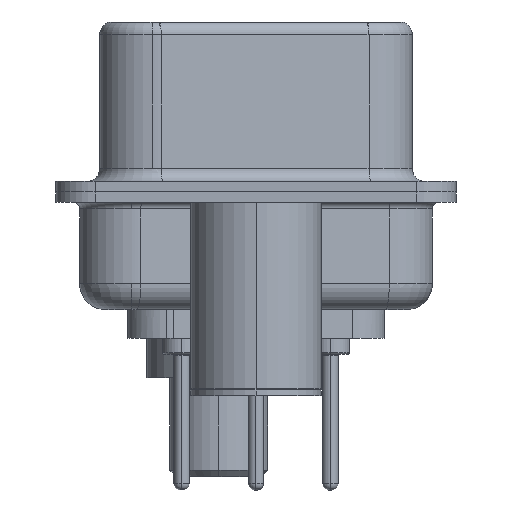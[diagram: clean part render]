
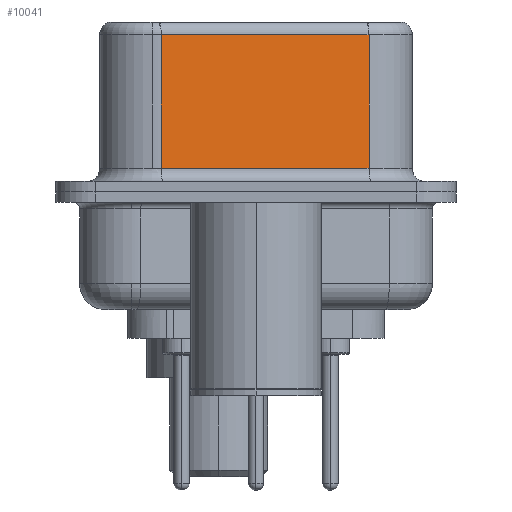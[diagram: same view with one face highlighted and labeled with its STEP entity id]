
A CAD part, left-side view. The second image highlights one B-rep face of the part: STEP entity #10041.
In plain terms, the highlighted planar face has unit normal (-0.985, -0.174, 0).
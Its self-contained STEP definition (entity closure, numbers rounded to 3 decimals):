
#919 = DIRECTION ( 'NONE',  ( 0.174, -0.985, 0. ) ) ;
#1303 = EDGE_CURVE ( 'NONE', #25222, #3450, #24702, .T. ) ;
#1446 = VERTEX_POINT ( 'NONE', #8338 ) ;
#1495 = AXIS2_PLACEMENT_3D ( 'NONE', #18260, #17339, #17264 ) ;
#2440 = VERTEX_POINT ( 'NONE', #22309 ) ;
#3299 = CARTESIAN_POINT ( 'NONE',  ( 5.132, -4.322, 0.9 ) ) ;
#3450 = VERTEX_POINT ( 'NONE', #3555 ) ;
#3555 = CARTESIAN_POINT ( 'NONE',  ( 3.73, 3.628, 0.9 ) ) ;
#4103 = LINE ( 'NONE', #16058, #23672 ) ;
#4176 = EDGE_CURVE ( 'NONE', #2440, #25222, #8430, .T. ) ;
#7643 = EDGE_CURVE ( 'NONE', #2440, #1446, #4103, .T. ) ;
#8153 = ORIENTED_EDGE ( 'NONE', *, *, #7643, .F. ) ;
#8338 = CARTESIAN_POINT ( 'NONE',  ( 5.132, -4.322, 0.9 ) ) ;
#8430 = LINE ( 'NONE', #15592, #13635 ) ;
#9150 = VECTOR ( 'NONE', #919, 1000. ) ;
#10041 = ADVANCED_FACE ( 'NONE', ( #12715 ), #17367, .F. ) ;
#10180 = DIRECTION ( 'NONE',  ( -0.174, 0.985, 0. ) ) ;
#10774 = DIRECTION ( 'NONE',  ( 0., 0., -1. ) ) ;
#11790 = CARTESIAN_POINT ( 'NONE',  ( 3.73, 3.628, 6.52 ) ) ;
#12318 = EDGE_CURVE ( 'NONE', #3450, #1446, #20375, .T. ) ;
#12715 = FACE_OUTER_BOUND ( 'NONE', #19303, .T. ) ;
#13635 = VECTOR ( 'NONE', #10180, 1000. ) ;
#13670 = CARTESIAN_POINT ( 'NONE',  ( 3.73, 3.628, 6.02 ) ) ;
#15592 = CARTESIAN_POINT ( 'NONE',  ( 5.132, -4.322, 6.02 ) ) ;
#16058 = CARTESIAN_POINT ( 'NONE',  ( 5.132, -4.322, 6.52 ) ) ;
#17264 = DIRECTION ( 'NONE',  ( -0.174, 0.985, 0. ) ) ;
#17339 = DIRECTION ( 'NONE',  ( 0.985, 0.174, 0. ) ) ;
#17367 = PLANE ( 'NONE',  #1495 ) ;
#18260 = CARTESIAN_POINT ( 'NONE',  ( 5.132, -4.322, 6.52 ) ) ;
#18634 = ORIENTED_EDGE ( 'NONE', *, *, #12318, .T. ) ;
#18743 = VECTOR ( 'NONE', #10774, 1000. ) ;
#19303 = EDGE_LOOP ( 'NONE', ( #8153, #25209, #28085, #18634 ) ) ;
#20375 = LINE ( 'NONE', #3299, #9150 ) ;
#22309 = CARTESIAN_POINT ( 'NONE',  ( 5.132, -4.322, 6.02 ) ) ;
#23672 = VECTOR ( 'NONE', #25100, 1000. ) ;
#24702 = LINE ( 'NONE', #11790, #18743 ) ;
#25100 = DIRECTION ( 'NONE',  ( 0., 0., -1. ) ) ;
#25209 = ORIENTED_EDGE ( 'NONE', *, *, #4176, .T. ) ;
#25222 = VERTEX_POINT ( 'NONE', #13670 ) ;
#28085 = ORIENTED_EDGE ( 'NONE', *, *, #1303, .T. ) ;
